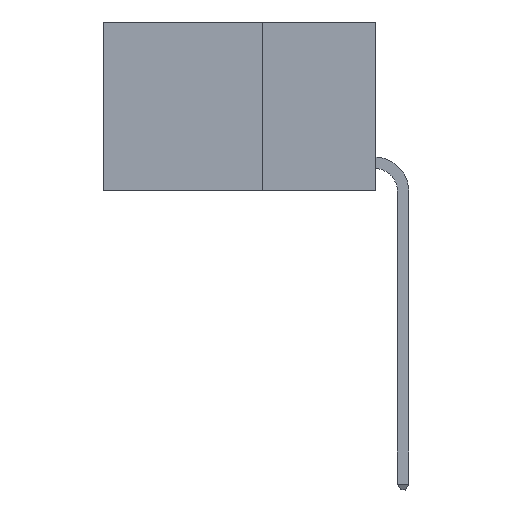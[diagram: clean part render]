
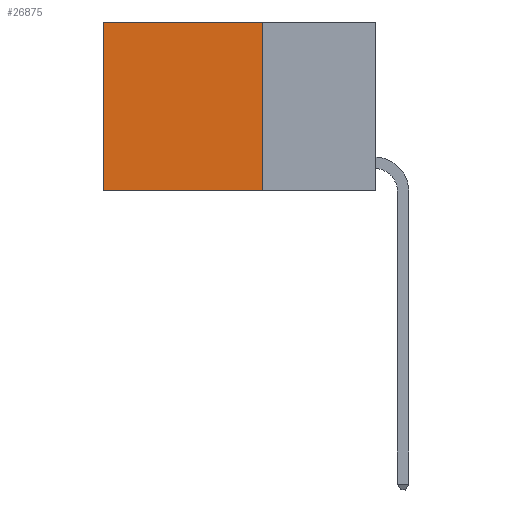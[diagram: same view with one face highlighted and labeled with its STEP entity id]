
A CAD part, left-side view. The second image highlights one B-rep face of the part: STEP entity #26875.
In plain terms, the highlighted planar face has unit normal (-1, 0, 0).
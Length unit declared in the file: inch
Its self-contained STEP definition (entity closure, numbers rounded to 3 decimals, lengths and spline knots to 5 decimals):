
#143 = CARTESIAN_POINT ( 'NONE',  ( 0.2625, 0.25, 0. ) ) ;
#296 = CARTESIAN_POINT ( 'NONE',  ( 0.2625, 0.6, 0. ) ) ;
#1342 = EDGE_CURVE ( 'NONE', #6960, #19977, #11989, .T. ) ;
#2647 = CARTESIAN_POINT ( 'NONE',  ( 0.2625, 0.6, 0. ) ) ;
#3082 = ORIENTED_EDGE ( 'NONE', *, *, #26897, .T. ) ;
#3219 = LINE ( 'NONE', #13723, #9522 ) ;
#4803 = EDGE_CURVE ( 'NONE', #20331, #6960, #3219, .T. ) ;
#4959 = DIRECTION ( 'NONE',  ( 0., 0., -1. ) ) ;
#5068 = DIRECTION ( 'NONE',  ( 0., 0., -1. ) ) ;
#5773 = VERTEX_POINT ( 'NONE', #296 ) ;
#6960 = VERTEX_POINT ( 'NONE', #22105 ) ;
#6993 = EDGE_CURVE ( 'NONE', #20331, #5773, #9031, .T. ) ;
#7451 = VECTOR ( 'NONE', #5068, 39.37008 ) ;
#8291 = VECTOR ( 'NONE', #26691, 39.37008 ) ;
#8894 = EDGE_LOOP ( 'NONE', ( #3082, #20808, #12941, #26797 ) ) ;
#9031 = LINE ( 'NONE', #19927, #8291 ) ;
#9522 = VECTOR ( 'NONE', #13730, 39.37008 ) ;
#11270 = VECTOR ( 'NONE', #27687, 39.37008 ) ;
#11989 = LINE ( 'NONE', #26011, #11270 ) ;
#12941 = ORIENTED_EDGE ( 'NONE', *, *, #4803, .F. ) ;
#13723 = CARTESIAN_POINT ( 'NONE',  ( 0.2625, 0.25, 0. ) ) ;
#13730 = DIRECTION ( 'NONE',  ( 0., 0., -1. ) ) ;
#14263 = PLANE ( 'NONE',  #20446 ) ;
#15727 = CARTESIAN_POINT ( 'NONE',  ( 0.2625, 0.6, -0.37 ) ) ;
#18886 = DIRECTION ( 'NONE',  ( 1., 0., 0. ) ) ;
#19927 = CARTESIAN_POINT ( 'NONE',  ( 0.2625, 0.25, 0. ) ) ;
#19977 = VERTEX_POINT ( 'NONE', #15727 ) ;
#20331 = VERTEX_POINT ( 'NONE', #28250 ) ;
#20446 = AXIS2_PLACEMENT_3D ( 'NONE', #143, #18886, #4959 ) ;
#20808 = ORIENTED_EDGE ( 'NONE', *, *, #1342, .F. ) ;
#21194 = FACE_OUTER_BOUND ( 'NONE', #8894, .T. ) ;
#22105 = CARTESIAN_POINT ( 'NONE',  ( 0.2625, 0.25, -0.37 ) ) ;
#25817 = LINE ( 'NONE', #2647, #7451 ) ;
#26011 = CARTESIAN_POINT ( 'NONE',  ( 0.2625, 0.25, -0.37 ) ) ;
#26691 = DIRECTION ( 'NONE',  ( 0., 1., 0. ) ) ;
#26797 = ORIENTED_EDGE ( 'NONE', *, *, #6993, .T. ) ;
#26875 = ADVANCED_FACE ( 'NONE', ( #21194 ), #14263, .F. ) ;
#26897 = EDGE_CURVE ( 'NONE', #5773, #19977, #25817, .T. ) ;
#27687 = DIRECTION ( 'NONE',  ( 0., 1., 0. ) ) ;
#28250 = CARTESIAN_POINT ( 'NONE',  ( 0.2625, 0.25, 0. ) ) ;
